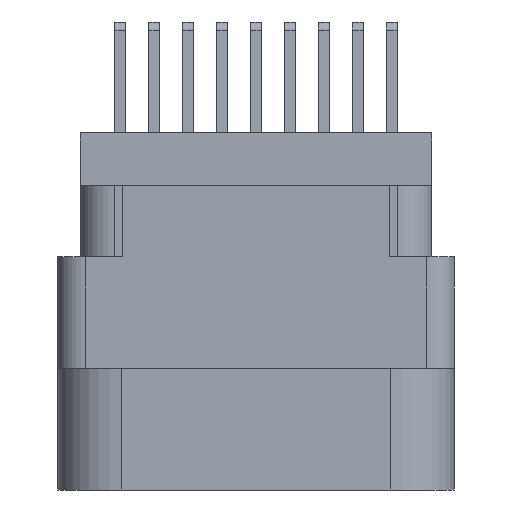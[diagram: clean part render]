
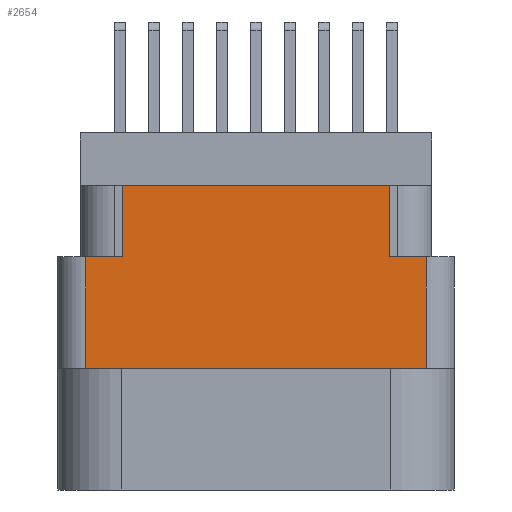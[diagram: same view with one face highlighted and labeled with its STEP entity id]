
A CAD part, left-side view. The second image highlights one B-rep face of the part: STEP entity #2654.
In plain terms, the highlighted planar face has unit normal (-1, 0, 0).
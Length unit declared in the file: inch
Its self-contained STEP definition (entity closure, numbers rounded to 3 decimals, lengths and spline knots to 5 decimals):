
#706 = EDGE_LOOP ( 'NONE', ( #9758, #24158, #33805, #3677, #12244, #22831, #8156, #5598 ) ) ;
#2654 = ADVANCED_FACE ( 'NONE', ( #32095 ), #13492, .T. ) ;
#3677 = ORIENTED_EDGE ( 'NONE', *, *, #43247, .T. ) ;
#4090 = LINE ( 'NONE', #4987, #11758 ) ;
#4302 = LINE ( 'NONE', #32152, #26296 ) ;
#4987 = CARTESIAN_POINT ( 'NONE',  ( -1.2955, 0.438, -0.117 ) ) ;
#5192 = VECTOR ( 'NONE', #21619, 39.37008 ) ;
#5598 = ORIENTED_EDGE ( 'NONE', *, *, #11101, .F. ) ;
#6894 = CARTESIAN_POINT ( 'NONE',  ( -1.2955, -0.296, -0.274 ) ) ;
#7312 = VERTEX_POINT ( 'NONE', #41976 ) ;
#7577 = CARTESIAN_POINT ( 'NONE',  ( -1.2955, 0., -0.52 ) ) ;
#8156 = ORIENTED_EDGE ( 'NONE', *, *, #40115, .F. ) ;
#8254 = CARTESIAN_POINT ( 'NONE',  ( -1.2955, -0.376, -0.52 ) ) ;
#8401 = DIRECTION ( 'NONE',  ( 0., 0., -1. ) ) ;
#9268 = CARTESIAN_POINT ( 'NONE',  ( -1.2955, -0.296, -0.274 ) ) ;
#9658 = CARTESIAN_POINT ( 'NONE',  ( -1.2955, 0.376, -0.274 ) ) ;
#9758 = ORIENTED_EDGE ( 'NONE', *, *, #42653, .F. ) ;
#10024 = DIRECTION ( 'NONE',  ( 0., 0., 1. ) ) ;
#10317 = EDGE_CURVE ( 'NONE', #20692, #35398, #15224, .T. ) ;
#11101 = EDGE_CURVE ( 'NONE', #34879, #7312, #4302, .T. ) ;
#11180 = CARTESIAN_POINT ( 'NONE',  ( -1.2955, 0.376, -0.789 ) ) ;
#11758 = VECTOR ( 'NONE', #39740, 39.37008 ) ;
#12244 = ORIENTED_EDGE ( 'NONE', *, *, #10317, .F. ) ;
#12375 = VECTOR ( 'NONE', #15010, 39.37008 ) ;
#13492 = PLANE ( 'NONE',  #28080 ) ;
#13612 = VERTEX_POINT ( 'NONE', #8254 ) ;
#13642 = EDGE_CURVE ( 'NONE', #13612, #29303, #42535, .T. ) ;
#15010 = DIRECTION ( 'NONE',  ( 0., -1., 0. ) ) ;
#15224 = LINE ( 'NONE', #22163, #12375 ) ;
#16458 = VECTOR ( 'NONE', #27837, 39.37008 ) ;
#16624 = CARTESIAN_POINT ( 'NONE',  ( -1.2955, -0.296, -0.117 ) ) ;
#17703 = LINE ( 'NONE', #6894, #16458 ) ;
#20692 = VERTEX_POINT ( 'NONE', #9268 ) ;
#21619 = DIRECTION ( 'NONE',  ( 0., 1., 0. ) ) ;
#22163 = CARTESIAN_POINT ( 'NONE',  ( -1.2955, 0., -0.274 ) ) ;
#22831 = ORIENTED_EDGE ( 'NONE', *, *, #31931, .T. ) ;
#24158 = ORIENTED_EDGE ( 'NONE', *, *, #43202, .T. ) ;
#24802 = CARTESIAN_POINT ( 'NONE',  ( -1.2955, 0., -0.274 ) ) ;
#25653 = DIRECTION ( 'NONE',  ( 0., 0., 1. ) ) ;
#26296 = VECTOR ( 'NONE', #28725, 39.37008 ) ;
#26349 = VERTEX_POINT ( 'NONE', #16624 ) ;
#27535 = CARTESIAN_POINT ( 'NONE',  ( -1.2955, -0.438, -0.789 ) ) ;
#27837 = DIRECTION ( 'NONE',  ( 0., 0., 1. ) ) ;
#28080 = AXIS2_PLACEMENT_3D ( 'NONE', #27535, #41548, #10024 ) ;
#28669 = LINE ( 'NONE', #35764, #29256 ) ;
#28725 = DIRECTION ( 'NONE',  ( 0., 0., 1. ) ) ;
#29102 = LINE ( 'NONE', #11180, #35135 ) ;
#29256 = VECTOR ( 'NONE', #25653, 39.37008 ) ;
#29303 = VERTEX_POINT ( 'NONE', #30613 ) ;
#30613 = CARTESIAN_POINT ( 'NONE',  ( -1.2955, 0.376, -0.52 ) ) ;
#31261 = DIRECTION ( 'NONE',  ( 0., -1., 0. ) ) ;
#31931 = EDGE_CURVE ( 'NONE', #20692, #26349, #17703, .T. ) ;
#32095 = FACE_OUTER_BOUND ( 'NONE', #706, .T. ) ;
#32152 = CARTESIAN_POINT ( 'NONE',  ( -1.2955, 0.296, -0.274 ) ) ;
#33369 = CARTESIAN_POINT ( 'NONE',  ( -1.2955, 0.296, -0.274 ) ) ;
#33763 = CARTESIAN_POINT ( 'NONE',  ( -1.2955, -0.376, -0.274 ) ) ;
#33805 = ORIENTED_EDGE ( 'NONE', *, *, #13642, .F. ) ;
#34879 = VERTEX_POINT ( 'NONE', #33369 ) ;
#35135 = VECTOR ( 'NONE', #8401, 39.37008 ) ;
#35154 = LINE ( 'NONE', #24802, #37284 ) ;
#35398 = VERTEX_POINT ( 'NONE', #33763 ) ;
#35764 = CARTESIAN_POINT ( 'NONE',  ( -1.2955, -0.376, -0.789 ) ) ;
#37284 = VECTOR ( 'NONE', #31261, 39.37008 ) ;
#39740 = DIRECTION ( 'NONE',  ( 0., -1., 0. ) ) ;
#40115 = EDGE_CURVE ( 'NONE', #7312, #26349, #4090, .T. ) ;
#41030 = VERTEX_POINT ( 'NONE', #9658 ) ;
#41548 = DIRECTION ( 'NONE',  ( -1., 0., 0. ) ) ;
#41976 = CARTESIAN_POINT ( 'NONE',  ( -1.2955, 0.296, -0.117 ) ) ;
#42535 = LINE ( 'NONE', #7577, #5192 ) ;
#42653 = EDGE_CURVE ( 'NONE', #41030, #34879, #35154, .T. ) ;
#43202 = EDGE_CURVE ( 'NONE', #41030, #29303, #29102, .T. ) ;
#43247 = EDGE_CURVE ( 'NONE', #13612, #35398, #28669, .T. ) ;
